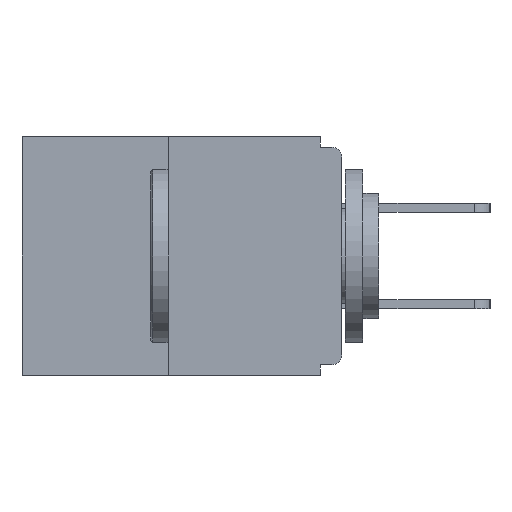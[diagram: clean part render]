
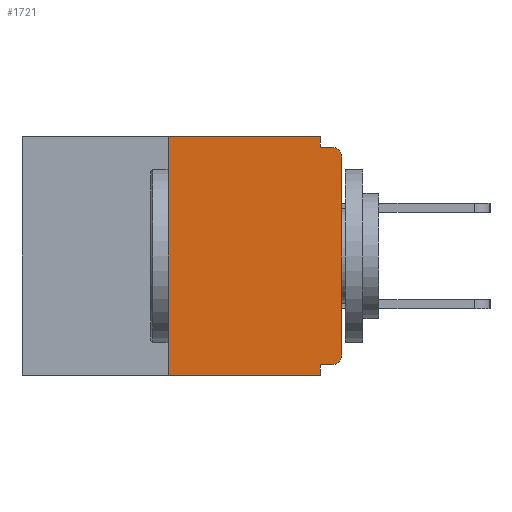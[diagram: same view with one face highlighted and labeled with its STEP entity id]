
A CAD part, left-side view. The second image highlights one B-rep face of the part: STEP entity #1721.
In plain terms, the highlighted planar face has unit normal (-1, 0, 0).
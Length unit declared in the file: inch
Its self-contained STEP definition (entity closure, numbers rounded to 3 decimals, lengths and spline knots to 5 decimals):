
#220 = EDGE_CURVE ( 'NONE', #17613, #16328, #12927, .T. ) ;
#754 = DIRECTION ( 'NONE',  ( 0., 0., -1. ) ) ;
#1409 = DIRECTION ( 'NONE',  ( 0., 0., -1. ) ) ;
#1697 = CARTESIAN_POINT ( 'NONE',  ( 0., 0., 0. ) ) ;
#1721 = ADVANCED_FACE ( 'NONE', ( #8655 ), #14443, .F. ) ;
#1937 = LINE ( 'NONE', #10393, #2828 ) ;
#2407 = CIRCLE ( 'NONE', #16464, 0.015 ) ;
#2828 = VECTOR ( 'NONE', #10721, 39.37008 ) ;
#3170 = EDGE_LOOP ( 'NONE', ( #9473, #7974, #6770, #5545, #5755, #15601, #4824, #4813, #16164, #13550 ) ) ;
#3276 = CARTESIAN_POINT ( 'NONE',  ( 0., 0.031, -0.328 ) ) ;
#3645 = CARTESIAN_POINT ( 'NONE',  ( 0., 0.031, 0. ) ) ;
#3917 = CARTESIAN_POINT ( 'NONE',  ( 0., 0.031, -0.343 ) ) ;
#4074 = DIRECTION ( 'NONE',  ( 0., 1., 0. ) ) ;
#4306 = CARTESIAN_POINT ( 'NONE',  ( 0., 0.46, 0. ) ) ;
#4430 = DIRECTION ( 'NONE',  ( 0., -1., 0. ) ) ;
#4575 = EDGE_CURVE ( 'NONE', #17613, #6456, #14352, .T. ) ;
#4764 = DIRECTION ( 'NONE',  ( 0., 0., 1. ) ) ;
#4813 = ORIENTED_EDGE ( 'NONE', *, *, #14697, .T. ) ;
#4824 = ORIENTED_EDGE ( 'NONE', *, *, #17554, .T. ) ;
#4825 = AXIS2_PLACEMENT_3D ( 'NONE', #10724, #17893, #13780 ) ;
#4883 = DIRECTION ( 'NONE',  ( 0., -1., 0. ) ) ;
#5191 = EDGE_CURVE ( 'NONE', #5707, #6456, #14768, .T. ) ;
#5201 = LINE ( 'NONE', #1697, #13061 ) ;
#5378 = VECTOR ( 'NONE', #4074, 39.37008 ) ;
#5545 = ORIENTED_EDGE ( 'NONE', *, *, #5191, .F. ) ;
#5707 = VERTEX_POINT ( 'NONE', #3276 ) ;
#5755 = ORIENTED_EDGE ( 'NONE', *, *, #13039, .F. ) ;
#5837 = VERTEX_POINT ( 'NONE', #7867 ) ;
#5844 = LINE ( 'NONE', #4306, #16850 ) ;
#6285 = EDGE_CURVE ( 'NONE', #11282, #7759, #1937, .T. ) ;
#6317 = CARTESIAN_POINT ( 'NONE',  ( 0., 0.25, 0. ) ) ;
#6456 = VERTEX_POINT ( 'NONE', #3917 ) ;
#6640 = VECTOR ( 'NONE', #11328, 39.37008 ) ;
#6734 = LINE ( 'NONE', #12554, #5378 ) ;
#6770 = ORIENTED_EDGE ( 'NONE', *, *, #4575, .T. ) ;
#7467 = VECTOR ( 'NONE', #754, 39.37008 ) ;
#7759 = VERTEX_POINT ( 'NONE', #16959 ) ;
#7867 = CARTESIAN_POINT ( 'NONE',  ( 0., 0., -0.313 ) ) ;
#7905 = CARTESIAN_POINT ( 'NONE',  ( 0., 0.031, -0.015 ) ) ;
#7974 = ORIENTED_EDGE ( 'NONE', *, *, #220, .F. ) ;
#7984 = DIRECTION ( 'NONE',  ( -1., 0., 0. ) ) ;
#8339 = EDGE_CURVE ( 'NONE', #13149, #5837, #8867, .T. ) ;
#8505 = CARTESIAN_POINT ( 'NONE',  ( 0., 0.25, 0. ) ) ;
#8573 = CARTESIAN_POINT ( 'NONE',  ( 0., 0.46, 0. ) ) ;
#8655 = FACE_OUTER_BOUND ( 'NONE', #3170, .T. ) ;
#8867 = CIRCLE ( 'NONE', #4825, 0.015 ) ;
#9111 = EDGE_CURVE ( 'NONE', #11000, #11282, #13059, .T. ) ;
#9473 = ORIENTED_EDGE ( 'NONE', *, *, #10592, .F. ) ;
#9627 = DIRECTION ( 'NONE',  ( 0., 0., -1. ) ) ;
#9895 = DIRECTION ( 'NONE',  ( 1., 0., 0. ) ) ;
#10393 = CARTESIAN_POINT ( 'NONE',  ( 0., 0., -0.015 ) ) ;
#10592 = EDGE_CURVE ( 'NONE', #16328, #11000, #5844, .T. ) ;
#10721 = DIRECTION ( 'NONE',  ( 0., -1., 0. ) ) ;
#10724 = CARTESIAN_POINT ( 'NONE',  ( 0., 0.015, -0.313 ) ) ;
#11000 = VERTEX_POINT ( 'NONE', #13969 ) ;
#11246 = AXIS2_PLACEMENT_3D ( 'NONE', #8573, #9895, #1409 ) ;
#11282 = VERTEX_POINT ( 'NONE', #7905 ) ;
#11328 = DIRECTION ( 'NONE',  ( 0., 0., 1. ) ) ;
#12048 = CARTESIAN_POINT ( 'NONE',  ( 0., 0., -0.03 ) ) ;
#12554 = CARTESIAN_POINT ( 'NONE',  ( 0., 0., -0.328 ) ) ;
#12927 = LINE ( 'NONE', #8505, #6640 ) ;
#13039 = EDGE_CURVE ( 'NONE', #13149, #5707, #6734, .T. ) ;
#13059 = LINE ( 'NONE', #3645, #7467 ) ;
#13061 = VECTOR ( 'NONE', #4764, 39.37008 ) ;
#13149 = VERTEX_POINT ( 'NONE', #14224 ) ;
#13367 = CARTESIAN_POINT ( 'NONE',  ( 0., 0.46, -0.343 ) ) ;
#13550 = ORIENTED_EDGE ( 'NONE', *, *, #9111, .F. ) ;
#13780 = DIRECTION ( 'NONE',  ( 0., 0., -1. ) ) ;
#13969 = CARTESIAN_POINT ( 'NONE',  ( 0., 0.031, 0. ) ) ;
#14066 = VERTEX_POINT ( 'NONE', #12048 ) ;
#14224 = CARTESIAN_POINT ( 'NONE',  ( 0., 0.015, -0.328 ) ) ;
#14352 = LINE ( 'NONE', #13367, #16382 ) ;
#14443 = PLANE ( 'NONE',  #11246 ) ;
#14680 = CARTESIAN_POINT ( 'NONE',  ( 0., 0.25, -0.343 ) ) ;
#14697 = EDGE_CURVE ( 'NONE', #14066, #7759, #2407, .T. ) ;
#14768 = LINE ( 'NONE', #16359, #16120 ) ;
#15601 = ORIENTED_EDGE ( 'NONE', *, *, #8339, .T. ) ;
#16120 = VECTOR ( 'NONE', #17824, 39.37008 ) ;
#16164 = ORIENTED_EDGE ( 'NONE', *, *, #6285, .F. ) ;
#16328 = VERTEX_POINT ( 'NONE', #6317 ) ;
#16359 = CARTESIAN_POINT ( 'NONE',  ( 0., 0.031, -0.343 ) ) ;
#16382 = VECTOR ( 'NONE', #4883, 39.37008 ) ;
#16464 = AXIS2_PLACEMENT_3D ( 'NONE', #16563, #7984, #9627 ) ;
#16563 = CARTESIAN_POINT ( 'NONE',  ( 0., 0.015, -0.03 ) ) ;
#16850 = VECTOR ( 'NONE', #4430, 39.37008 ) ;
#16959 = CARTESIAN_POINT ( 'NONE',  ( 0., 0.015, -0.015 ) ) ;
#17554 = EDGE_CURVE ( 'NONE', #5837, #14066, #5201, .T. ) ;
#17613 = VERTEX_POINT ( 'NONE', #14680 ) ;
#17824 = DIRECTION ( 'NONE',  ( 0., 0., -1. ) ) ;
#17893 = DIRECTION ( 'NONE',  ( -1., 0., 0. ) ) ;
